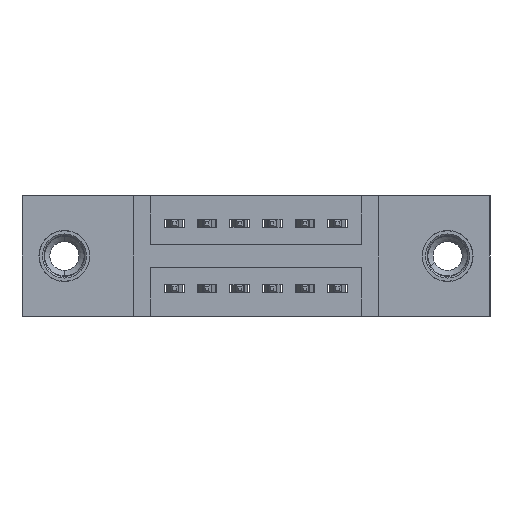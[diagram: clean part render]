
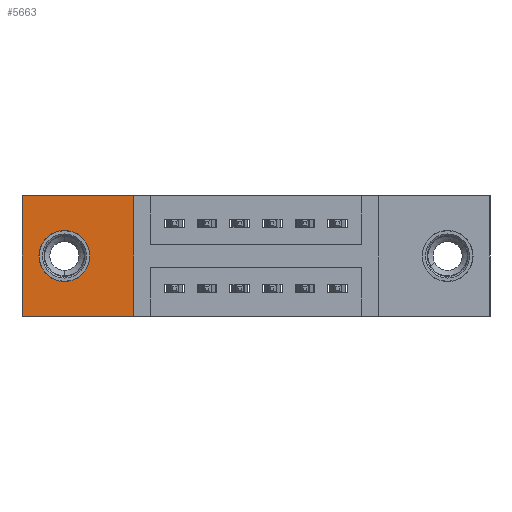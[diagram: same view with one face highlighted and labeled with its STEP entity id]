
A CAD part, front view. The second image highlights one B-rep face of the part: STEP entity #5663.
In plain terms, the highlighted planar face has unit normal (0, -1, 0).
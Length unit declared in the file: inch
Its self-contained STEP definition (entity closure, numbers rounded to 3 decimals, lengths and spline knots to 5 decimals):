
#49 = VECTOR ( 'NONE', #2007, 39.37008 ) ;
#116 = DIRECTION ( 'NONE',  ( 0., 0., -1. ) ) ;
#366 = DIRECTION ( 'NONE',  ( 0., -1., 0. ) ) ;
#951 = CARTESIAN_POINT ( 'NONE',  ( 0., 0.11, 0. ) ) ;
#1085 = ORIENTED_EDGE ( 'NONE', *, *, #7817, .T. ) ;
#1169 = DIRECTION ( 'NONE',  ( 1., 0., 0. ) ) ;
#1297 = PLANE ( 'NONE',  #9390 ) ;
#1505 = CARTESIAN_POINT ( 'NONE',  ( 0., 0.11, -0.37 ) ) ;
#1523 = EDGE_LOOP ( 'NONE', ( #6003, #1085, #2521, #5528 ) ) ;
#1602 = FACE_BOUND ( 'NONE', #3886, .T. ) ;
#1919 = CARTESIAN_POINT ( 'NONE',  ( 0.13, 0.11, -0.263 ) ) ;
#2007 = DIRECTION ( 'NONE',  ( -1., 0., 0. ) ) ;
#2336 = VECTOR ( 'NONE', #5942, 39.37008 ) ;
#2447 = LINE ( 'NONE', #10553, #7696 ) ;
#2452 = LINE ( 'NONE', #4790, #2336 ) ;
#2513 = LINE ( 'NONE', #8024, #49 ) ;
#2521 = ORIENTED_EDGE ( 'NONE', *, *, #6385, .T. ) ;
#3498 = ORIENTED_EDGE ( 'NONE', *, *, #8414, .F. ) ;
#3571 = EDGE_CURVE ( 'NONE', #10724, #8637, #2513, .T. ) ;
#3846 = CIRCLE ( 'NONE', #4293, 0.078 ) ;
#3886 = EDGE_LOOP ( 'NONE', ( #9028, #3498 ) ) ;
#3926 = VERTEX_POINT ( 'NONE', #1505 ) ;
#3946 = CARTESIAN_POINT ( 'NONE',  ( 0.3425, 0.11, -0.37 ) ) ;
#4293 = AXIS2_PLACEMENT_3D ( 'NONE', #10537, #5410, #7996 ) ;
#4394 = CARTESIAN_POINT ( 'NONE',  ( 0.3425, 0.11, 0. ) ) ;
#4591 = FACE_OUTER_BOUND ( 'NONE', #1523, .T. ) ;
#4790 = CARTESIAN_POINT ( 'NONE',  ( 0.3425, 0.11, 0. ) ) ;
#5410 = DIRECTION ( 'NONE',  ( 0., -1., 0. ) ) ;
#5528 = ORIENTED_EDGE ( 'NONE', *, *, #3571, .T. ) ;
#5663 = ADVANCED_FACE ( 'NONE', ( #1602, #4591 ), #1297, .T. ) ;
#5942 = DIRECTION ( 'NONE',  ( 0., 0., 1. ) ) ;
#6003 = ORIENTED_EDGE ( 'NONE', *, *, #6399, .T. ) ;
#6208 = CARTESIAN_POINT ( 'NONE',  ( 0.13, 0.11, -0.185 ) ) ;
#6232 = DIRECTION ( 'NONE',  ( 0., -1., 0. ) ) ;
#6385 = EDGE_CURVE ( 'NONE', #6660, #10724, #2452, .T. ) ;
#6399 = EDGE_CURVE ( 'NONE', #8637, #3926, #9706, .T. ) ;
#6410 = CARTESIAN_POINT ( 'NONE',  ( 0., 0.11, 0. ) ) ;
#6660 = VERTEX_POINT ( 'NONE', #3946 ) ;
#7187 = VECTOR ( 'NONE', #116, 39.37008 ) ;
#7684 = CIRCLE ( 'NONE', #9722, 0.078 ) ;
#7696 = VECTOR ( 'NONE', #1169, 39.37008 ) ;
#7817 = EDGE_CURVE ( 'NONE', #3926, #6660, #2447, .T. ) ;
#7870 = VERTEX_POINT ( 'NONE', #10677 ) ;
#7996 = DIRECTION ( 'NONE',  ( 0., 0., -1. ) ) ;
#8024 = CARTESIAN_POINT ( 'NONE',  ( 0., 0.11, 0. ) ) ;
#8414 = EDGE_CURVE ( 'NONE', #10382, #7870, #7684, .T. ) ;
#8637 = VERTEX_POINT ( 'NONE', #6410 ) ;
#8691 = DIRECTION ( 'NONE',  ( 0., 0., -1. ) ) ;
#8748 = DIRECTION ( 'NONE',  ( 0., 0., -1. ) ) ;
#9016 = EDGE_CURVE ( 'NONE', #7870, #10382, #3846, .T. ) ;
#9028 = ORIENTED_EDGE ( 'NONE', *, *, #9016, .F. ) ;
#9390 = AXIS2_PLACEMENT_3D ( 'NONE', #9567, #6232, #8691 ) ;
#9567 = CARTESIAN_POINT ( 'NONE',  ( 0., 0.11, -0.37 ) ) ;
#9706 = LINE ( 'NONE', #951, #7187 ) ;
#9722 = AXIS2_PLACEMENT_3D ( 'NONE', #6208, #366, #8748 ) ;
#10382 = VERTEX_POINT ( 'NONE', #1919 ) ;
#10537 = CARTESIAN_POINT ( 'NONE',  ( 0.13, 0.11, -0.185 ) ) ;
#10553 = CARTESIAN_POINT ( 'NONE',  ( 0., 0.11, -0.37 ) ) ;
#10677 = CARTESIAN_POINT ( 'NONE',  ( 0.13, 0.11, -0.107 ) ) ;
#10724 = VERTEX_POINT ( 'NONE', #4394 ) ;
